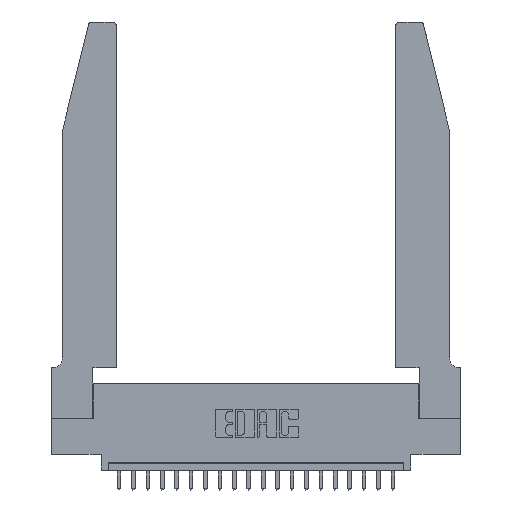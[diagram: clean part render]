
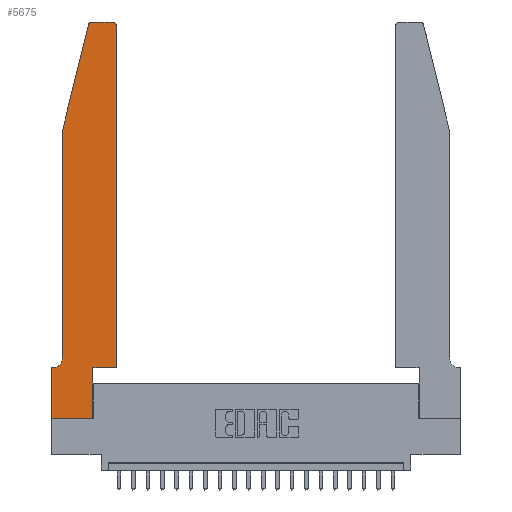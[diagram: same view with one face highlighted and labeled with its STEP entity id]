
A CAD part, top view. The second image highlights one B-rep face of the part: STEP entity #5675.
In plain terms, the highlighted planar face has unit normal (0, 0, 1).
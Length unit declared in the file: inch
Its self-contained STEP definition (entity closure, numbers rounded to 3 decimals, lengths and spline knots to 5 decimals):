
#5 = CARTESIAN_POINT ( 'NONE',  ( 0., 0., 0.37 ) ) ;
#62 = CARTESIAN_POINT ( 'NONE',  ( 0.2605, 2.75, 0.37 ) ) ;
#340 = CIRCLE ( 'NONE', #6410, 0.07 ) ;
#379 = EDGE_CURVE ( 'NONE', #15938, #6517, #12819, .T. ) ;
#428 = CARTESIAN_POINT ( 'NONE',  ( 0., 0.35, 0.37 ) ) ;
#448 = VECTOR ( 'NONE', #20339, 39.37008 ) ;
#683 = EDGE_CURVE ( 'NONE', #3150, #7550, #2856, .T. ) ;
#713 = CARTESIAN_POINT ( 'NONE',  ( 0.25487, 2.72718, 0.37 ) ) ;
#1104 = EDGE_CURVE ( 'NONE', #17339, #15938, #7276, .T. ) ;
#1214 = VECTOR ( 'NONE', #8735, 39.37008 ) ;
#1647 = EDGE_LOOP ( 'NONE', ( #5322, #6307, #17169, #8293, #15867, #2514, #14441, #12229, #21762, #21382, #2158, #13572 ) ) ;
#1761 = CARTESIAN_POINT ( 'NONE',  ( 0.284, 2.75, 0.37 ) ) ;
#2158 = ORIENTED_EDGE ( 'NONE', *, *, #19420, .T. ) ;
#2363 = PLANE ( 'NONE',  #6720 ) ;
#2514 = ORIENTED_EDGE ( 'NONE', *, *, #7352, .T. ) ;
#2575 = VECTOR ( 'NONE', #22245, 39.37008 ) ;
#2666 = DIRECTION ( 'NONE',  ( 0., 1., 0. ) ) ;
#2856 = LINE ( 'NONE', #5, #15555 ) ;
#3150 = VERTEX_POINT ( 'NONE', #8935 ) ;
#3263 = CARTESIAN_POINT ( 'NONE',  ( 0., 0.35, 0.37 ) ) ;
#4487 = CARTESIAN_POINT ( 'NONE',  ( 0.2865, 0., 0.37 ) ) ;
#4519 = CARTESIAN_POINT ( 'NONE',  ( 0.4505, 0.35, 0.37 ) ) ;
#4591 = DIRECTION ( 'NONE',  ( 0., 0., 1. ) ) ;
#4601 = LINE ( 'NONE', #7940, #448 ) ;
#4793 = VECTOR ( 'NONE', #6213, 39.37008 ) ;
#5322 = ORIENTED_EDGE ( 'NONE', *, *, #5801, .T. ) ;
#5647 = EDGE_CURVE ( 'NONE', #6517, #8236, #340, .T. ) ;
#5675 = ADVANCED_FACE ( 'NONE', ( #13588 ), #2363, .T. ) ;
#5746 = VERTEX_POINT ( 'NONE', #4519 ) ;
#5801 = EDGE_CURVE ( 'NONE', #7963, #6112, #13292, .T. ) ;
#5988 = DIRECTION ( 'NONE',  ( 1., 0., 0. ) ) ;
#6112 = VERTEX_POINT ( 'NONE', #1761 ) ;
#6213 = DIRECTION ( 'NONE',  ( -1., 0., 0. ) ) ;
#6307 = ORIENTED_EDGE ( 'NONE', *, *, #12318, .T. ) ;
#6410 = AXIS2_PLACEMENT_3D ( 'NONE', #18135, #16463, #7769 ) ;
#6517 = VERTEX_POINT ( 'NONE', #19989 ) ;
#6720 = AXIS2_PLACEMENT_3D ( 'NONE', #428, #12976, #11086 ) ;
#6775 = DIRECTION ( 'NONE',  ( 1., 0., 0. ) ) ;
#7276 = LINE ( 'NONE', #15095, #2575 ) ;
#7352 = EDGE_CURVE ( 'NONE', #8236, #13510, #15173, .T. ) ;
#7546 = CARTESIAN_POINT ( 'NONE',  ( 0.2865, 0.35, 0.37 ) ) ;
#7550 = VERTEX_POINT ( 'NONE', #4487 ) ;
#7769 = DIRECTION ( 'NONE',  ( -1., 0., 0. ) ) ;
#7898 = CIRCLE ( 'NONE', #15836, 0.03 ) ;
#7940 = CARTESIAN_POINT ( 'NONE',  ( 0., 0., 0.37 ) ) ;
#7963 = VERTEX_POINT ( 'NONE', #12315 ) ;
#8236 = VERTEX_POINT ( 'NONE', #15751 ) ;
#8293 = ORIENTED_EDGE ( 'NONE', *, *, #379, .T. ) ;
#8603 = CARTESIAN_POINT ( 'NONE',  ( 0.0755, 2., 0.37 ) ) ;
#8735 = DIRECTION ( 'NONE',  ( 0., -1., 0. ) ) ;
#8809 = DIRECTION ( 'NONE',  ( 0., 1., 0. ) ) ;
#8935 = CARTESIAN_POINT ( 'NONE',  ( 0., 0., 0.37 ) ) ;
#9746 = LINE ( 'NONE', #19405, #15530 ) ;
#9916 = DIRECTION ( 'NONE',  ( -1., 0., 0. ) ) ;
#11086 = DIRECTION ( 'NONE',  ( 1., 0., 0. ) ) ;
#11515 = DIRECTION ( 'NONE',  ( 1., 0., 0. ) ) ;
#11793 = VERTEX_POINT ( 'NONE', #17626 ) ;
#11863 = VECTOR ( 'NONE', #9916, 39.37008 ) ;
#11995 = EDGE_CURVE ( 'NONE', #13510, #3150, #4601, .T. ) ;
#12229 = ORIENTED_EDGE ( 'NONE', *, *, #683, .T. ) ;
#12315 = CARTESIAN_POINT ( 'NONE',  ( 0.4205, 2.75, 0.37 ) ) ;
#12318 = EDGE_CURVE ( 'NONE', #6112, #17339, #7898, .T. ) ;
#12819 = LINE ( 'NONE', #18855, #1214 ) ;
#12976 = DIRECTION ( 'NONE',  ( 0., 0., 1. ) ) ;
#13149 = LINE ( 'NONE', #22436, #22043 ) ;
#13292 = LINE ( 'NONE', #62, #4793 ) ;
#13510 = VERTEX_POINT ( 'NONE', #3263 ) ;
#13536 = DIRECTION ( 'NONE',  ( 1., 0., 0. ) ) ;
#13572 = ORIENTED_EDGE ( 'NONE', *, *, #16348, .T. ) ;
#13588 = FACE_OUTER_BOUND ( 'NONE', #1647, .T. ) ;
#13924 = VERTEX_POINT ( 'NONE', #16481 ) ;
#14441 = ORIENTED_EDGE ( 'NONE', *, *, #11995, .T. ) ;
#15095 = CARTESIAN_POINT ( 'NONE',  ( 0.0755, 2., 0.37 ) ) ;
#15132 = CARTESIAN_POINT ( 'NONE',  ( 0.4205, 2.72, 0.37 ) ) ;
#15173 = LINE ( 'NONE', #17075, #11863 ) ;
#15530 = VECTOR ( 'NONE', #8809, 39.37008 ) ;
#15555 = VECTOR ( 'NONE', #13536, 39.37008 ) ;
#15751 = CARTESIAN_POINT ( 'NONE',  ( 0.0055, 0.35, 0.37 ) ) ;
#15836 = AXIS2_PLACEMENT_3D ( 'NONE', #22550, #22470, #6775 ) ;
#15867 = ORIENTED_EDGE ( 'NONE', *, *, #5647, .T. ) ;
#15938 = VERTEX_POINT ( 'NONE', #8603 ) ;
#16348 = EDGE_CURVE ( 'NONE', #11793, #7963, #19858, .T. ) ;
#16463 = DIRECTION ( 'NONE',  ( 0., 0., -1. ) ) ;
#16481 = CARTESIAN_POINT ( 'NONE',  ( 0.2865, 0.35, 0.37 ) ) ;
#16619 = EDGE_CURVE ( 'NONE', #13924, #5746, #13149, .T. ) ;
#17075 = CARTESIAN_POINT ( 'NONE',  ( 0.0755, 0.35, 0.37 ) ) ;
#17169 = ORIENTED_EDGE ( 'NONE', *, *, #1104, .T. ) ;
#17339 = VERTEX_POINT ( 'NONE', #713 ) ;
#17626 = CARTESIAN_POINT ( 'NONE',  ( 0.4505, 2.72, 0.37 ) ) ;
#17752 = LINE ( 'NONE', #7546, #22177 ) ;
#18135 = CARTESIAN_POINT ( 'NONE',  ( 0.0055, 0.42, 0.37 ) ) ;
#18855 = CARTESIAN_POINT ( 'NONE',  ( 0.0755, 2., 0.37 ) ) ;
#19405 = CARTESIAN_POINT ( 'NONE',  ( 0.4505, 0.35, 0.37 ) ) ;
#19420 = EDGE_CURVE ( 'NONE', #5746, #11793, #9746, .T. ) ;
#19466 = AXIS2_PLACEMENT_3D ( 'NONE', #15132, #4591, #5988 ) ;
#19858 = CIRCLE ( 'NONE', #19466, 0.03 ) ;
#19868 = EDGE_CURVE ( 'NONE', #7550, #13924, #17752, .T. ) ;
#19989 = CARTESIAN_POINT ( 'NONE',  ( 0.0755, 0.42, 0.37 ) ) ;
#20339 = DIRECTION ( 'NONE',  ( 0., -1., 0. ) ) ;
#21382 = ORIENTED_EDGE ( 'NONE', *, *, #16619, .T. ) ;
#21762 = ORIENTED_EDGE ( 'NONE', *, *, #19868, .T. ) ;
#22043 = VECTOR ( 'NONE', #11515, 39.37008 ) ;
#22177 = VECTOR ( 'NONE', #2666, 39.37008 ) ;
#22245 = DIRECTION ( 'NONE',  ( -0.239, -0.971, 0. ) ) ;
#22436 = CARTESIAN_POINT ( 'NONE',  ( 0.4505, 0.35, 0.37 ) ) ;
#22470 = DIRECTION ( 'NONE',  ( 0., 0., 1. ) ) ;
#22550 = CARTESIAN_POINT ( 'NONE',  ( 0.284, 2.72, 0.37 ) ) ;
